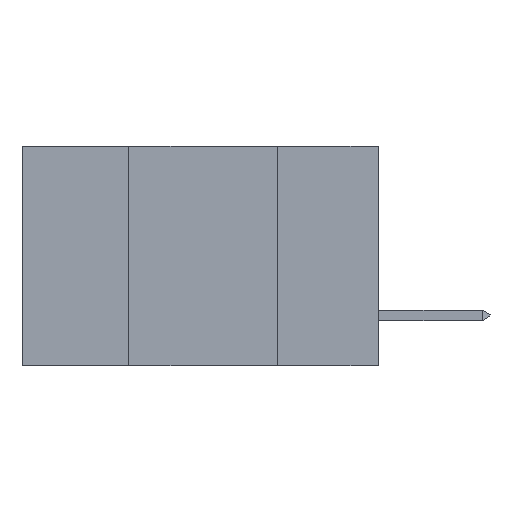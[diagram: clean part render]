
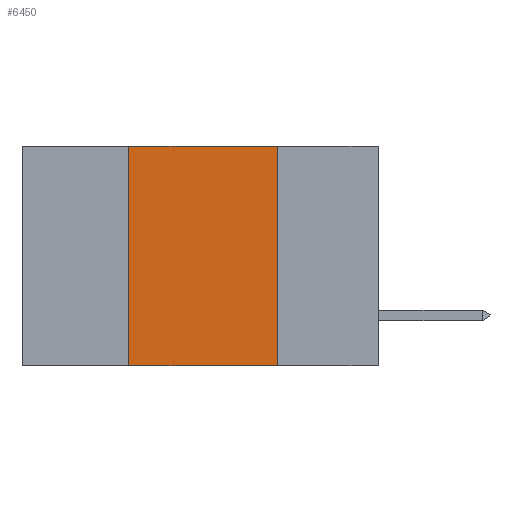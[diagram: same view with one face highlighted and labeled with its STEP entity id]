
A CAD part, left-side view. The second image highlights one B-rep face of the part: STEP entity #6450.
In plain terms, the highlighted planar face has unit normal (-1, 0, 0).
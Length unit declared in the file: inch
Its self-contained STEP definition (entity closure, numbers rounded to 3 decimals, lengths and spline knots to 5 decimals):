
#601 = DIRECTION ( 'NONE',  ( 1., 0., 0. ) ) ;
#639 = CARTESIAN_POINT ( 'NONE',  ( 0., 0.17, 0. ) ) ;
#1631 = VERTEX_POINT ( 'NONE', #13431 ) ;
#1855 = CARTESIAN_POINT ( 'NONE',  ( 0., 0.6, 0. ) ) ;
#2815 = EDGE_CURVE ( 'NONE', #11757, #1631, #5907, .T. ) ;
#3000 = FACE_OUTER_BOUND ( 'NONE', #14555, .T. ) ;
#3356 = ORIENTED_EDGE ( 'NONE', *, *, #13134, .F. ) ;
#3535 = LINE ( 'NONE', #4707, #14137 ) ;
#3603 = DIRECTION ( 'NONE',  ( 0., -1., 0. ) ) ;
#4374 = VECTOR ( 'NONE', #3603, 39.37008 ) ;
#4707 = CARTESIAN_POINT ( 'NONE',  ( 0., 0.42, -0.37 ) ) ;
#4829 = VECTOR ( 'NONE', #14905, 39.37008 ) ;
#5689 = AXIS2_PLACEMENT_3D ( 'NONE', #1855, #601, #6557 ) ;
#5907 = LINE ( 'NONE', #10852, #4374 ) ;
#6361 = ORIENTED_EDGE ( 'NONE', *, *, #12244, .F. ) ;
#6450 = ADVANCED_FACE ( 'NONE', ( #3000 ), #13393, .F. ) ;
#6519 = LINE ( 'NONE', #11383, #4829 ) ;
#6557 = DIRECTION ( 'NONE',  ( 0., 0., -1. ) ) ;
#9238 = EDGE_CURVE ( 'NONE', #11757, #11689, #3535, .T. ) ;
#9406 = DIRECTION ( 'NONE',  ( 0., 0., 1. ) ) ;
#9584 = VERTEX_POINT ( 'NONE', #639 ) ;
#9594 = LINE ( 'NONE', #14704, #12173 ) ;
#10852 = CARTESIAN_POINT ( 'NONE',  ( 0., 0.6, -0.37 ) ) ;
#11383 = CARTESIAN_POINT ( 'NONE',  ( 0., 0.17, -0.37 ) ) ;
#11689 = VERTEX_POINT ( 'NONE', #14290 ) ;
#11757 = VERTEX_POINT ( 'NONE', #13503 ) ;
#12173 = VECTOR ( 'NONE', #14349, 39.37008 ) ;
#12244 = EDGE_CURVE ( 'NONE', #11689, #9584, #9594, .T. ) ;
#13134 = EDGE_CURVE ( 'NONE', #9584, #1631, #6519, .T. ) ;
#13393 = PLANE ( 'NONE',  #5689 ) ;
#13431 = CARTESIAN_POINT ( 'NONE',  ( 0., 0.17, -0.37 ) ) ;
#13503 = CARTESIAN_POINT ( 'NONE',  ( 0., 0.42, -0.37 ) ) ;
#14137 = VECTOR ( 'NONE', #9406, 39.37008 ) ;
#14290 = CARTESIAN_POINT ( 'NONE',  ( 0., 0.42, 0. ) ) ;
#14349 = DIRECTION ( 'NONE',  ( 0., -1., 0. ) ) ;
#14408 = ORIENTED_EDGE ( 'NONE', *, *, #9238, .F. ) ;
#14454 = ORIENTED_EDGE ( 'NONE', *, *, #2815, .T. ) ;
#14555 = EDGE_LOOP ( 'NONE', ( #3356, #6361, #14408, #14454 ) ) ;
#14704 = CARTESIAN_POINT ( 'NONE',  ( 0., 0.6, 0. ) ) ;
#14905 = DIRECTION ( 'NONE',  ( 0., 0., -1. ) ) ;
